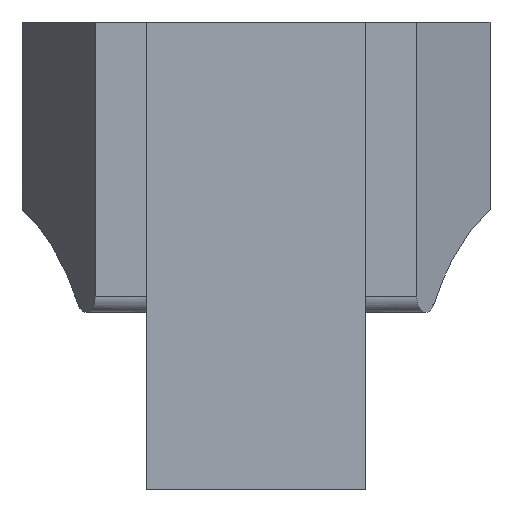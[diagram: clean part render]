
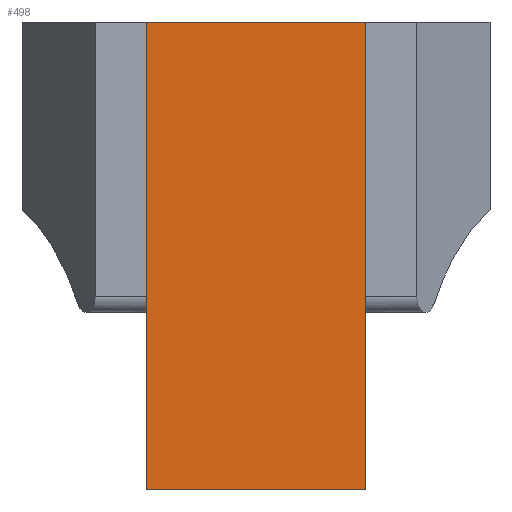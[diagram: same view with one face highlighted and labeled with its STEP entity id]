
A CAD part, front view. The second image highlights one B-rep face of the part: STEP entity #498.
In plain terms, the highlighted planar face has unit normal (0, -1, 0).
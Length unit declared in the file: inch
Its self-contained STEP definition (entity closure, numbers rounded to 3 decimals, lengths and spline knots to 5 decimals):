
#4 = EDGE_CURVE ( 'NONE', #237, #872, #488, .T. ) ;
#21 = CARTESIAN_POINT ( 'NONE',  ( 0.3458, -1.448, -1.475 ) ) ;
#51 = DIRECTION ( 'NONE',  ( 0., 0., -1. ) ) ;
#95 = EDGE_LOOP ( 'NONE', ( #218, #154, #1580, #662 ) ) ;
#97 = EDGE_CURVE ( 'NONE', #237, #367, #359, .T. ) ;
#120 = VECTOR ( 'NONE', #829, 39.37008 ) ;
#154 = ORIENTED_EDGE ( 'NONE', *, *, #97, .F. ) ;
#218 = ORIENTED_EDGE ( 'NONE', *, *, #1283, .F. ) ;
#237 = VERTEX_POINT ( 'NONE', #1662 ) ;
#238 = CARTESIAN_POINT ( 'NONE',  ( 0.3458, -1.448, -1.475 ) ) ;
#295 = DIRECTION ( 'NONE',  ( 0., 0., 1. ) ) ;
#298 = DIRECTION ( 'NONE',  ( 1., 0., 0. ) ) ;
#304 = AXIS2_PLACEMENT_3D ( 'NONE', #459, #862, #51 ) ;
#359 = LINE ( 'NONE', #462, #671 ) ;
#367 = VERTEX_POINT ( 'NONE', #1299 ) ;
#439 = FACE_OUTER_BOUND ( 'NONE', #95, .T. ) ;
#459 = CARTESIAN_POINT ( 'NONE',  ( 0.3458, -1.448, -1.475 ) ) ;
#462 = CARTESIAN_POINT ( 'NONE',  ( -0.3458, -1.448, -1.475 ) ) ;
#488 = LINE ( 'NONE', #238, #120 ) ;
#494 = VECTOR ( 'NONE', #298, 39.37008 ) ;
#498 = ADVANCED_FACE ( 'NONE', ( #439 ), #1636, .T. ) ;
#662 = ORIENTED_EDGE ( 'NONE', *, *, #877, .T. ) ;
#671 = VECTOR ( 'NONE', #1123, 39.37008 ) ;
#829 = DIRECTION ( 'NONE',  ( 1., 0., 0. ) ) ;
#841 = LINE ( 'NONE', #1232, #494 ) ;
#862 = DIRECTION ( 'NONE',  ( 0., -1., 0. ) ) ;
#872 = VERTEX_POINT ( 'NONE', #21 ) ;
#877 = EDGE_CURVE ( 'NONE', #872, #1287, #1115, .T. ) ;
#962 = CARTESIAN_POINT ( 'NONE',  ( 0.3458, -1.448, -1.475 ) ) ;
#1115 = LINE ( 'NONE', #962, #1459 ) ;
#1123 = DIRECTION ( 'NONE',  ( 0., 0., 1. ) ) ;
#1232 = CARTESIAN_POINT ( 'NONE',  ( 0.3458, -1.448, 0. ) ) ;
#1283 = EDGE_CURVE ( 'NONE', #367, #1287, #841, .T. ) ;
#1287 = VERTEX_POINT ( 'NONE', #1616 ) ;
#1299 = CARTESIAN_POINT ( 'NONE',  ( -0.3458, -1.448, 0. ) ) ;
#1459 = VECTOR ( 'NONE', #295, 39.37008 ) ;
#1580 = ORIENTED_EDGE ( 'NONE', *, *, #4, .T. ) ;
#1616 = CARTESIAN_POINT ( 'NONE',  ( 0.3458, -1.448, 0. ) ) ;
#1636 = PLANE ( 'NONE',  #304 ) ;
#1662 = CARTESIAN_POINT ( 'NONE',  ( -0.3458, -1.448, -1.475 ) ) ;
